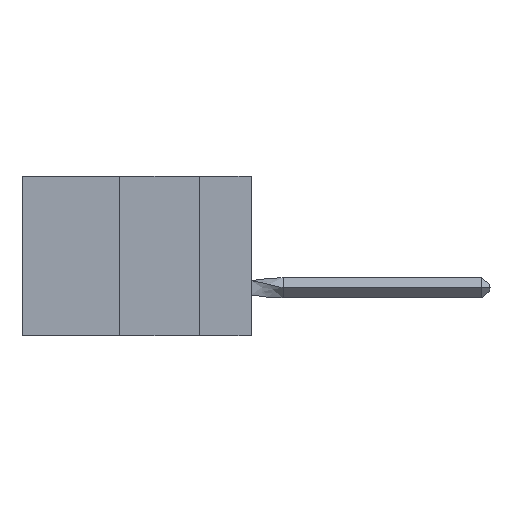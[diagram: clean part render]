
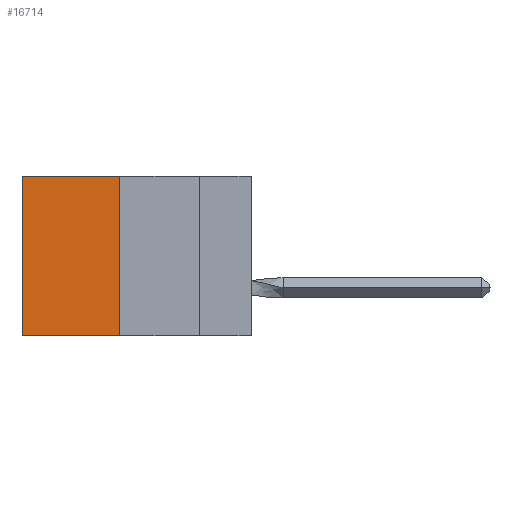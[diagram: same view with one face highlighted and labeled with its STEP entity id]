
A CAD part, left-side view. The second image highlights one B-rep face of the part: STEP entity #16714.
In plain terms, the highlighted planar face has unit normal (-1, 0, 0).
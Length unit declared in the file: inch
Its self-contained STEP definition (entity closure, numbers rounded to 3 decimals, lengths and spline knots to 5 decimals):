
#387 = CARTESIAN_POINT ( 'NONE',  ( 0.305, 0.413, 0. ) ) ;
#656 = CARTESIAN_POINT ( 'NONE',  ( 0.305, 0.413, -0.5 ) ) ;
#711 = EDGE_CURVE ( 'NONE', #1115, #24080, #15203, .T. ) ;
#941 = FACE_OUTER_BOUND ( 'NONE', #6836, .T. ) ;
#1115 = VERTEX_POINT ( 'NONE', #6604 ) ;
#3062 = DIRECTION ( 'NONE',  ( 0., 0., -1. ) ) ;
#3441 = EDGE_CURVE ( 'NONE', #24080, #13027, #19828, .T. ) ;
#4422 = CARTESIAN_POINT ( 'NONE',  ( 0.305, 0.413, -0.5 ) ) ;
#4671 = VECTOR ( 'NONE', #11154, 39.37008 ) ;
#5272 = VECTOR ( 'NONE', #3062, 39.37008 ) ;
#6604 = CARTESIAN_POINT ( 'NONE',  ( 0.305, 0.413, 0. ) ) ;
#6836 = EDGE_LOOP ( 'NONE', ( #16035, #11210, #24035, #20262 ) ) ;
#6909 = VECTOR ( 'NONE', #21089, 39.37008 ) ;
#7577 = CARTESIAN_POINT ( 'NONE',  ( 0.305, 0.72, 0. ) ) ;
#9261 = CARTESIAN_POINT ( 'NONE',  ( 0.305, 0.72, -0.5 ) ) ;
#11154 = DIRECTION ( 'NONE',  ( 0., 1., 0. ) ) ;
#11210 = ORIENTED_EDGE ( 'NONE', *, *, #12256, .F. ) ;
#11872 = AXIS2_PLACEMENT_3D ( 'NONE', #4422, #16750, #14661 ) ;
#12256 = EDGE_CURVE ( 'NONE', #12781, #13027, #23197, .T. ) ;
#12781 = VERTEX_POINT ( 'NONE', #656 ) ;
#13027 = VERTEX_POINT ( 'NONE', #9261 ) ;
#14491 = PLANE ( 'NONE',  #11872 ) ;
#14661 = DIRECTION ( 'NONE',  ( 0., 0., -1. ) ) ;
#15203 = LINE ( 'NONE', #387, #4671 ) ;
#15356 = VECTOR ( 'NONE', #21158, 39.37008 ) ;
#15552 = CARTESIAN_POINT ( 'NONE',  ( 0.305, 0.413, -0.5 ) ) ;
#16035 = ORIENTED_EDGE ( 'NONE', *, *, #3441, .T. ) ;
#16714 = ADVANCED_FACE ( 'NONE', ( #941 ), #14491, .F. ) ;
#16750 = DIRECTION ( 'NONE',  ( 1., 0., 0. ) ) ;
#17333 = CARTESIAN_POINT ( 'NONE',  ( 0.305, 0.72, -0.5 ) ) ;
#17409 = LINE ( 'NONE', #15552, #5272 ) ;
#19828 = LINE ( 'NONE', #17333, #15356 ) ;
#20262 = ORIENTED_EDGE ( 'NONE', *, *, #711, .T. ) ;
#21089 = DIRECTION ( 'NONE',  ( 0., 1., 0. ) ) ;
#21158 = DIRECTION ( 'NONE',  ( 0., 0., -1. ) ) ;
#23197 = LINE ( 'NONE', #23249, #6909 ) ;
#23249 = CARTESIAN_POINT ( 'NONE',  ( 0.305, 0.413, -0.5 ) ) ;
#24035 = ORIENTED_EDGE ( 'NONE', *, *, #26189, .F. ) ;
#24080 = VERTEX_POINT ( 'NONE', #7577 ) ;
#26189 = EDGE_CURVE ( 'NONE', #1115, #12781, #17409, .T. ) ;
